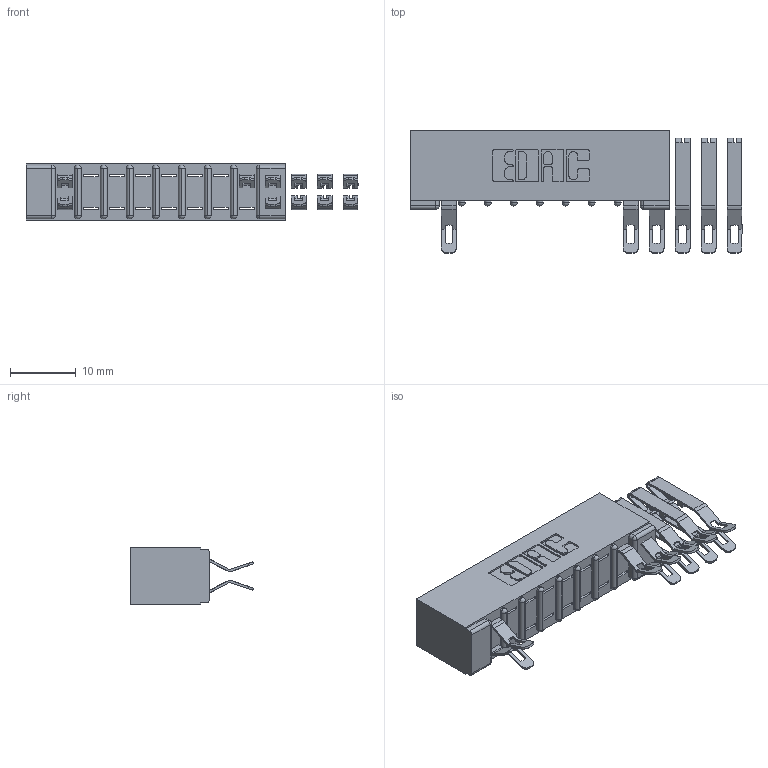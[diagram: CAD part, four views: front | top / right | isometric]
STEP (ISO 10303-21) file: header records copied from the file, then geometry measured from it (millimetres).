
FILE_DESCRIPTION (( 'STEP AP203' ), '1' );
FILE_NAME ('357-024-555-201.STEP', '2018-08-09T01:09:44', ( '' ), ( '' ), 'SwSTEP 2.0', 'SolidWorks 2016', '' );
FILE_SCHEMA (( 'CONFIG_CONTROL_DESIGN' ));
Length unit declared in the file: inch
Products named in the file (3): 307 Part_No Mounting Lugs; 307-290-001_555; 357-024-555-201
Assembly tree (12 placements, depth 2):
  357-024-555-201
    307 Part_No Mounting Lugs
    307-290-001_555  x11
Bounding box: 50.63 x 18.75 x 8.71 mm (x, y, z)
Volume: 2791.2 mm3; surface area: 4469.3 mm2
Topology: 12 solids, 12 shells, 840 faces, 2450 edges, 1592 vertices
Faces by surface type: plane 470, cylinder 352, sphere 18
Entity records: 11405 total; most frequent: CARTESIAN_POINT 1899, ORIENTED_EDGE 1884, DIRECTION 1876, EDGE_CURVE 942, LINE 698, VECTOR 698, VERTEX_POINT 612, AXIS2_PLACEMENT_3D 589
